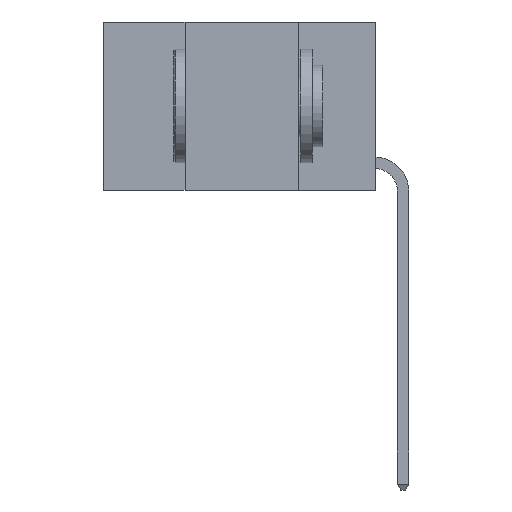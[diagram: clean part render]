
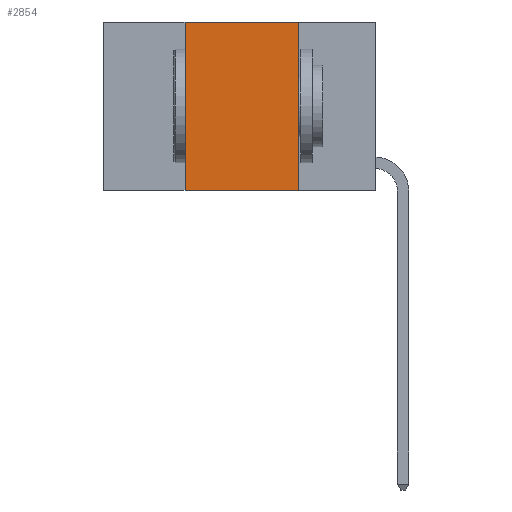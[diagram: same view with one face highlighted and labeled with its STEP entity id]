
A CAD part, left-side view. The second image highlights one B-rep face of the part: STEP entity #2854.
In plain terms, the highlighted planar face has unit normal (-1, 0, 0).
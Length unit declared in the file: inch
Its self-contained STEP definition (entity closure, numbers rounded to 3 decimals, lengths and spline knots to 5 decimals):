
#371 = CARTESIAN_POINT ( 'NONE',  ( 0., 0.42, 0. ) ) ;
#496 = CARTESIAN_POINT ( 'NONE',  ( 0., 0.17, 0. ) ) ;
#644 = EDGE_CURVE ( 'NONE', #3994, #1242, #1420, .T. ) ;
#1084 = CARTESIAN_POINT ( 'NONE',  ( 0., 0.42, -0.37 ) ) ;
#1143 = VECTOR ( 'NONE', #8107, 39.37008 ) ;
#1167 = VERTEX_POINT ( 'NONE', #1084 ) ;
#1175 = DIRECTION ( 'NONE',  ( 0., 0., -1. ) ) ;
#1242 = VERTEX_POINT ( 'NONE', #2966 ) ;
#1261 = VERTEX_POINT ( 'NONE', #2801 ) ;
#1266 = DIRECTION ( 'NONE',  ( 1., 0., 0. ) ) ;
#1319 = PLANE ( 'NONE',  #5921 ) ;
#1420 = LINE ( 'NONE', #1872, #8372 ) ;
#1675 = CARTESIAN_POINT ( 'NONE',  ( 0., 0.6, 0. ) ) ;
#1730 = EDGE_CURVE ( 'NONE', #1167, #1261, #6669, .T. ) ;
#1872 = CARTESIAN_POINT ( 'NONE',  ( 0., 0.6, 0. ) ) ;
#1938 = DIRECTION ( 'NONE',  ( 0., -1., 0. ) ) ;
#1944 = LINE ( 'NONE', #496, #8831 ) ;
#2099 = DIRECTION ( 'NONE',  ( 0., 0., -1. ) ) ;
#2231 = CARTESIAN_POINT ( 'NONE',  ( 0., 0.42, 0. ) ) ;
#2518 = VECTOR ( 'NONE', #3367, 39.37008 ) ;
#2801 = CARTESIAN_POINT ( 'NONE',  ( 0., 0.17, -0.37 ) ) ;
#2854 = ADVANCED_FACE ( 'NONE', ( #5827 ), #1319, .F. ) ;
#2966 = CARTESIAN_POINT ( 'NONE',  ( 0., 0.17, 0. ) ) ;
#3100 = EDGE_CURVE ( 'NONE', #1167, #3994, #4387, .T. ) ;
#3367 = DIRECTION ( 'NONE',  ( 0., 0., 1. ) ) ;
#3880 = EDGE_CURVE ( 'NONE', #1242, #1261, #1944, .T. ) ;
#3994 = VERTEX_POINT ( 'NONE', #2231 ) ;
#4387 = LINE ( 'NONE', #371, #2518 ) ;
#4663 = ORIENTED_EDGE ( 'NONE', *, *, #3100, .F. ) ;
#5130 = ORIENTED_EDGE ( 'NONE', *, *, #3880, .F. ) ;
#5827 = FACE_OUTER_BOUND ( 'NONE', #7049, .T. ) ;
#5921 = AXIS2_PLACEMENT_3D ( 'NONE', #1675, #1266, #1175 ) ;
#6669 = LINE ( 'NONE', #8922, #1143 ) ;
#6815 = ORIENTED_EDGE ( 'NONE', *, *, #644, .F. ) ;
#7049 = EDGE_LOOP ( 'NONE', ( #5130, #6815, #4663, #7907 ) ) ;
#7907 = ORIENTED_EDGE ( 'NONE', *, *, #1730, .T. ) ;
#8107 = DIRECTION ( 'NONE',  ( 0., -1., 0. ) ) ;
#8372 = VECTOR ( 'NONE', #1938, 39.37008 ) ;
#8831 = VECTOR ( 'NONE', #2099, 39.37008 ) ;
#8922 = CARTESIAN_POINT ( 'NONE',  ( 0., 0.6, -0.37 ) ) ;
